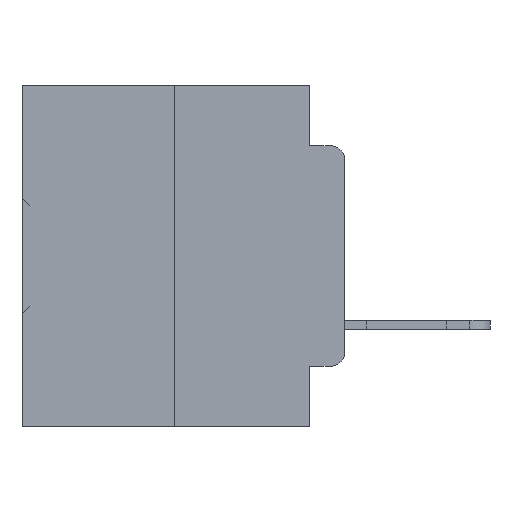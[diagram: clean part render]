
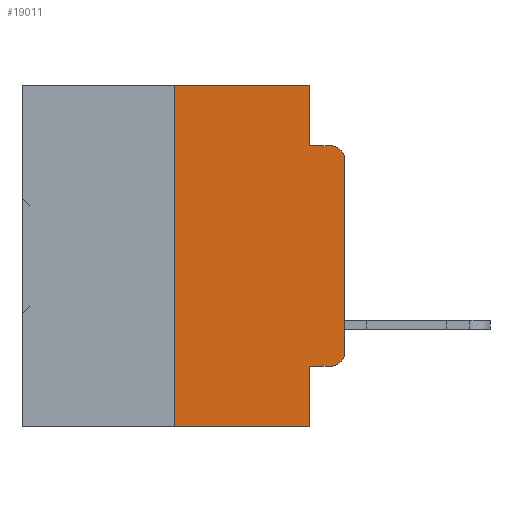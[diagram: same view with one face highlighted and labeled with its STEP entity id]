
A CAD part, left-side view. The second image highlights one B-rep face of the part: STEP entity #19011.
In plain terms, the highlighted planar face has unit normal (-1, 0, 0).
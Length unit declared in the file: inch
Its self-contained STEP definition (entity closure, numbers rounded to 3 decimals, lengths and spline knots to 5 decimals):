
#1502 = VECTOR ( 'NONE', #34112, 39.37008 ) ;
#1656 = VERTEX_POINT ( 'NONE', #7993 ) ;
#1906 = VERTEX_POINT ( 'NONE', #14919 ) ;
#2617 = ORIENTED_EDGE ( 'NONE', *, *, #31614, .T. ) ;
#2958 = DIRECTION ( 'NONE',  ( 0., -1., 0. ) ) ;
#3111 = ORIENTED_EDGE ( 'NONE', *, *, #19506, .F. ) ;
#3139 = CARTESIAN_POINT ( 'NONE',  ( 0., 0.051, -0.4115 ) ) ;
#4047 = LINE ( 'NONE', #35746, #26362 ) ;
#4587 = CARTESIAN_POINT ( 'NONE',  ( 0., 0.25, 0. ) ) ;
#4965 = VERTEX_POINT ( 'NONE', #19091 ) ;
#5945 = LINE ( 'NONE', #4587, #35543 ) ;
#6364 = VECTOR ( 'NONE', #13185, 39.37008 ) ;
#7198 = PLANE ( 'NONE',  #26848 ) ;
#7449 = VECTOR ( 'NONE', #2958, 39.37008 ) ;
#7671 = CARTESIAN_POINT ( 'NONE',  ( 0., 0.051, 0. ) ) ;
#7993 = CARTESIAN_POINT ( 'NONE',  ( 0., 0.25, -0.5 ) ) ;
#8062 = ORIENTED_EDGE ( 'NONE', *, *, #22194, .T. ) ;
#8339 = VERTEX_POINT ( 'NONE', #15051 ) ;
#9072 = VECTOR ( 'NONE', #10960, 39.37008 ) ;
#10533 = ORIENTED_EDGE ( 'NONE', *, *, #18818, .T. ) ;
#10649 = EDGE_CURVE ( 'NONE', #8339, #4965, #30187, .T. ) ;
#10797 = CARTESIAN_POINT ( 'NONE',  ( 0., 0.02, -0.3915 ) ) ;
#10960 = DIRECTION ( 'NONE',  ( 0., 0., 1. ) ) ;
#10966 = DIRECTION ( 'NONE',  ( 0., 0., 1. ) ) ;
#11077 = LINE ( 'NONE', #25842, #9072 ) ;
#13185 = DIRECTION ( 'NONE',  ( 0., -1., 0. ) ) ;
#13370 = CARTESIAN_POINT ( 'NONE',  ( 0., 0.051, 0. ) ) ;
#13555 = DIRECTION ( 'NONE',  ( 1., 0., 0. ) ) ;
#13991 = DIRECTION ( 'NONE',  ( 0., 0., -1. ) ) ;
#14823 = CARTESIAN_POINT ( 'NONE',  ( 0., 0.473, 0. ) ) ;
#14919 = CARTESIAN_POINT ( 'NONE',  ( 0., 0.02, -0.0885 ) ) ;
#15051 = CARTESIAN_POINT ( 'NONE',  ( 0., 0.25, 0. ) ) ;
#15294 = VERTEX_POINT ( 'NONE', #31383 ) ;
#15503 = ORIENTED_EDGE ( 'NONE', *, *, #20295, .F. ) ;
#15870 = DIRECTION ( 'NONE',  ( 0., -1., 0. ) ) ;
#16110 = CARTESIAN_POINT ( 'NONE',  ( 0., 0., -0.1085 ) ) ;
#16532 = AXIS2_PLACEMENT_3D ( 'NONE', #10797, #31362, #13991 ) ;
#16781 = CIRCLE ( 'NONE', #16532, 0.02 ) ;
#17829 = EDGE_LOOP ( 'NONE', ( #25564, #10533, #3111, #20796, #29044, #15503, #8062, #25988, #2617, #27757 ) ) ;
#18477 = EDGE_CURVE ( 'NONE', #18556, #30368, #11077, .T. ) ;
#18556 = VERTEX_POINT ( 'NONE', #34547 ) ;
#18818 = EDGE_CURVE ( 'NONE', #30368, #1906, #29489, .T. ) ;
#18945 = DIRECTION ( 'NONE',  ( -1., 0., 0. ) ) ;
#19011 = ADVANCED_FACE ( 'NONE', ( #20778 ), #7198, .F. ) ;
#19091 = CARTESIAN_POINT ( 'NONE',  ( 0., 0.051, 0. ) ) ;
#19506 = EDGE_CURVE ( 'NONE', #31315, #1906, #4047, .T. ) ;
#19675 = EDGE_CURVE ( 'NONE', #4965, #31315, #36865, .T. ) ;
#20295 = EDGE_CURVE ( 'NONE', #1656, #8339, #5945, .T. ) ;
#20432 = VERTEX_POINT ( 'NONE', #37680 ) ;
#20778 = FACE_OUTER_BOUND ( 'NONE', #17829, .T. ) ;
#20796 = ORIENTED_EDGE ( 'NONE', *, *, #19675, .F. ) ;
#21109 = CARTESIAN_POINT ( 'NONE',  ( 0., 0.02, -0.4115 ) ) ;
#21180 = VECTOR ( 'NONE', #25307, 39.37008 ) ;
#22194 = EDGE_CURVE ( 'NONE', #1656, #15294, #23720, .T. ) ;
#23720 = LINE ( 'NONE', #35595, #7449 ) ;
#25307 = DIRECTION ( 'NONE',  ( 0., 0., -1. ) ) ;
#25564 = ORIENTED_EDGE ( 'NONE', *, *, #18477, .T. ) ;
#25842 = CARTESIAN_POINT ( 'NONE',  ( 0., 0., 0. ) ) ;
#25953 = LINE ( 'NONE', #7671, #1502 ) ;
#25988 = ORIENTED_EDGE ( 'NONE', *, *, #33766, .F. ) ;
#26137 = LINE ( 'NONE', #3139, #32718 ) ;
#26362 = VECTOR ( 'NONE', #30191, 39.37008 ) ;
#26848 = AXIS2_PLACEMENT_3D ( 'NONE', #28148, #13555, #33784 ) ;
#27757 = ORIENTED_EDGE ( 'NONE', *, *, #36291, .T. ) ;
#28148 = CARTESIAN_POINT ( 'NONE',  ( 0., 0.473, 0. ) ) ;
#29044 = ORIENTED_EDGE ( 'NONE', *, *, #10649, .F. ) ;
#29397 = AXIS2_PLACEMENT_3D ( 'NONE', #35789, #18945, #38442 ) ;
#29489 = CIRCLE ( 'NONE', #29397, 0.02 ) ;
#29705 = VERTEX_POINT ( 'NONE', #21109 ) ;
#30187 = LINE ( 'NONE', #14823, #6364 ) ;
#30191 = DIRECTION ( 'NONE',  ( 0., -1., 0. ) ) ;
#30368 = VERTEX_POINT ( 'NONE', #16110 ) ;
#31315 = VERTEX_POINT ( 'NONE', #34645 ) ;
#31362 = DIRECTION ( 'NONE',  ( -1., 0., 0. ) ) ;
#31383 = CARTESIAN_POINT ( 'NONE',  ( 0., 0.051, -0.5 ) ) ;
#31614 = EDGE_CURVE ( 'NONE', #20432, #29705, #26137, .T. ) ;
#32718 = VECTOR ( 'NONE', #15870, 39.37008 ) ;
#33766 = EDGE_CURVE ( 'NONE', #20432, #15294, #25953, .T. ) ;
#33784 = DIRECTION ( 'NONE',  ( 0., 0., -1. ) ) ;
#34112 = DIRECTION ( 'NONE',  ( 0., 0., -1. ) ) ;
#34547 = CARTESIAN_POINT ( 'NONE',  ( 0., 0., -0.3915 ) ) ;
#34645 = CARTESIAN_POINT ( 'NONE',  ( 0., 0.051, -0.0885 ) ) ;
#35543 = VECTOR ( 'NONE', #10966, 39.37008 ) ;
#35595 = CARTESIAN_POINT ( 'NONE',  ( 0., 0.473, -0.5 ) ) ;
#35746 = CARTESIAN_POINT ( 'NONE',  ( 0., 0.051, -0.0885 ) ) ;
#35789 = CARTESIAN_POINT ( 'NONE',  ( 0., 0.02, -0.1085 ) ) ;
#36291 = EDGE_CURVE ( 'NONE', #29705, #18556, #16781, .T. ) ;
#36865 = LINE ( 'NONE', #13370, #21180 ) ;
#37680 = CARTESIAN_POINT ( 'NONE',  ( 0., 0.051, -0.4115 ) ) ;
#38442 = DIRECTION ( 'NONE',  ( 0., 0., -1. ) ) ;
